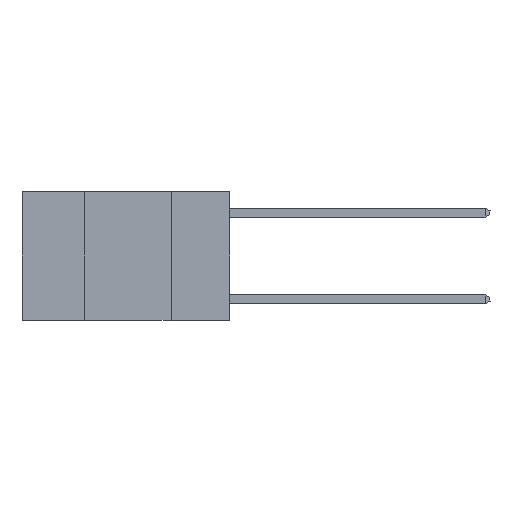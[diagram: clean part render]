
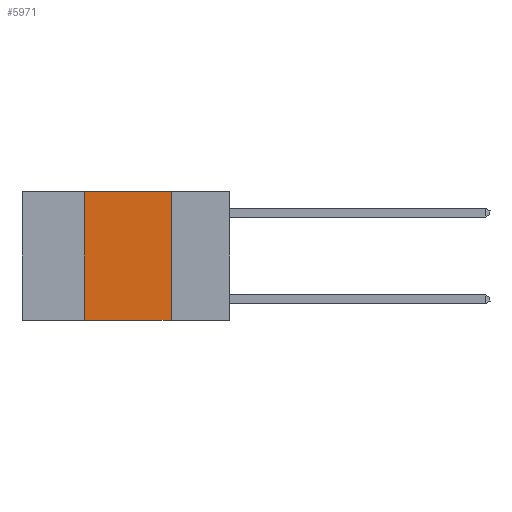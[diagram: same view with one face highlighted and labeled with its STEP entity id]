
A CAD part, left-side view. The second image highlights one B-rep face of the part: STEP entity #5971.
In plain terms, the highlighted planar face has unit normal (-1, 0, 0).
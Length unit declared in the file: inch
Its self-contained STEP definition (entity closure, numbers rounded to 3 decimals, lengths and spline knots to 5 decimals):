
#267 = DIRECTION ( 'NONE',  ( 0., 0., -1. ) ) ;
#640 = VERTEX_POINT ( 'NONE', #9730 ) ;
#2148 = DIRECTION ( 'NONE',  ( 0., -1., 0. ) ) ;
#2865 = ORIENTED_EDGE ( 'NONE', *, *, #8784, .F. ) ;
#4288 = CARTESIAN_POINT ( 'NONE',  ( 0., 0.42, 0. ) ) ;
#5234 = CARTESIAN_POINT ( 'NONE',  ( 0., 0.6, 0. ) ) ;
#5627 = CARTESIAN_POINT ( 'NONE',  ( 0., 0.17, -0.37 ) ) ;
#5642 = VECTOR ( 'NONE', #6110, 39.37008 ) ;
#5825 = EDGE_LOOP ( 'NONE', ( #26514, #2865, #9756, #15154 ) ) ;
#5971 = ADVANCED_FACE ( 'NONE', ( #17892 ), #11354, .F. ) ;
#6110 = DIRECTION ( 'NONE',  ( 0., 0., -1. ) ) ;
#8109 = VECTOR ( 'NONE', #18678, 39.37008 ) ;
#8262 = CARTESIAN_POINT ( 'NONE',  ( 0., 0.6, -0.37 ) ) ;
#8784 = EDGE_CURVE ( 'NONE', #24787, #27585, #16158, .T. ) ;
#9104 = EDGE_CURVE ( 'NONE', #640, #14178, #19473, .T. ) ;
#9461 = DIRECTION ( 'NONE',  ( 1., 0., 0. ) ) ;
#9730 = CARTESIAN_POINT ( 'NONE',  ( 0., 0.42, -0.37 ) ) ;
#9756 = ORIENTED_EDGE ( 'NONE', *, *, #10476, .F. ) ;
#10476 = EDGE_CURVE ( 'NONE', #640, #24787, #16917, .T. ) ;
#10492 = LINE ( 'NONE', #19367, #5642 ) ;
#11354 = PLANE ( 'NONE',  #23794 ) ;
#12558 = CARTESIAN_POINT ( 'NONE',  ( 0., 0.42, 0. ) ) ;
#12689 = VECTOR ( 'NONE', #14129, 39.37008 ) ;
#14129 = DIRECTION ( 'NONE',  ( 0., -1., 0. ) ) ;
#14178 = VERTEX_POINT ( 'NONE', #5627 ) ;
#15154 = ORIENTED_EDGE ( 'NONE', *, *, #9104, .T. ) ;
#16158 = LINE ( 'NONE', #5234, #12689 ) ;
#16917 = LINE ( 'NONE', #12558, #8109 ) ;
#17892 = FACE_OUTER_BOUND ( 'NONE', #5825, .T. ) ;
#18678 = DIRECTION ( 'NONE',  ( 0., 0., 1. ) ) ;
#19117 = EDGE_CURVE ( 'NONE', #27585, #14178, #10492, .T. ) ;
#19367 = CARTESIAN_POINT ( 'NONE',  ( 0., 0.17, 0. ) ) ;
#19473 = LINE ( 'NONE', #8262, #21534 ) ;
#19713 = CARTESIAN_POINT ( 'NONE',  ( 0., 0.17, 0. ) ) ;
#20233 = CARTESIAN_POINT ( 'NONE',  ( 0., 0.6, 0. ) ) ;
#21534 = VECTOR ( 'NONE', #2148, 39.37008 ) ;
#23794 = AXIS2_PLACEMENT_3D ( 'NONE', #20233, #9461, #267 ) ;
#24787 = VERTEX_POINT ( 'NONE', #4288 ) ;
#26514 = ORIENTED_EDGE ( 'NONE', *, *, #19117, .F. ) ;
#27585 = VERTEX_POINT ( 'NONE', #19713 ) ;
